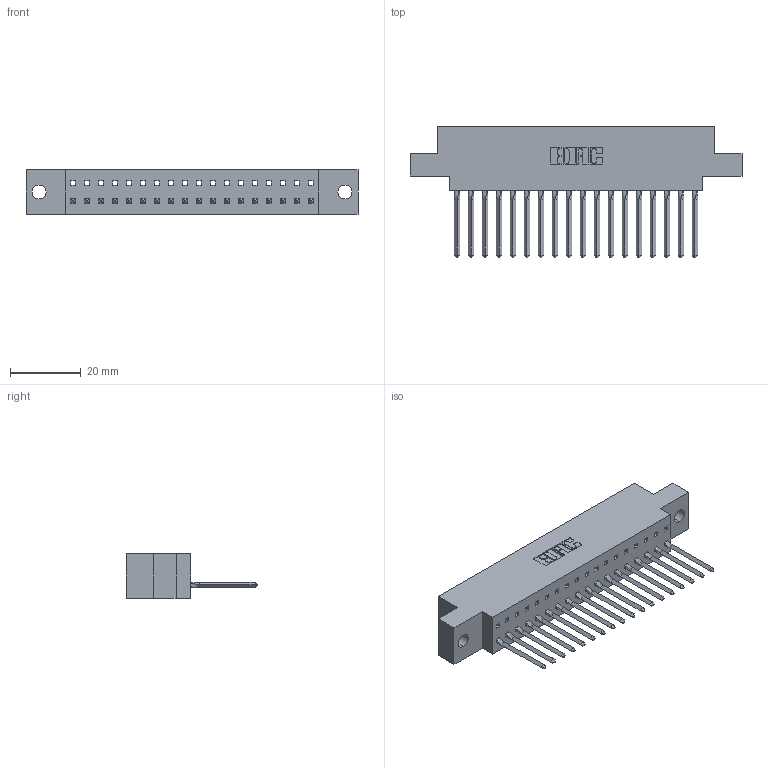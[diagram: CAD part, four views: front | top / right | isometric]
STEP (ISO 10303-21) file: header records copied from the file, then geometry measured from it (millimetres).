
FILE_DESCRIPTION (( 'STEP AP203' ), '1' );
FILE_NAME ('317-018-542-604.STEP', '2020-02-27T15:49:21', ( '' ), ( '' ), 'SwSTEP 2.0', 'SolidWorks 2016', '' );
FILE_SCHEMA (( 'CONFIG_CONTROL_DESIGN' ));
Length unit declared in the file: inch
Products named in the file (3): 317-018-542-604; 317 Part_.156 Dia - TH; 317-290-003_542
Assembly tree (19 placements, depth 2):
  317-018-542-604
    317 Part_.156 Dia - TH
    317-290-003_542  x18
Bounding box: 94.03 x 37.34 x 12.7 mm (x, y, z)
Volume: 13799.2 mm3; surface area: 16099.6 mm2
Topology: 19 solids, 19 shells, 1452 faces, 4181 edges, 2702 vertices
Faces by surface type: plane 1210, cylinder 170, bspline 72
Entity records: 27811 total; most frequent: CARTESIAN_POINT 5179, ORIENTED_EDGE 4860, DIRECTION 4094, EDGE_CURVE 2430, LINE 2260, VECTOR 2260, VERTEX_POINT 1614, AXIS2_PLACEMENT_3D 917
